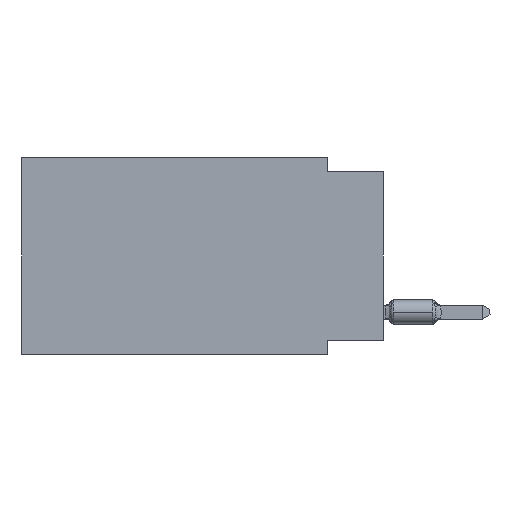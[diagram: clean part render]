
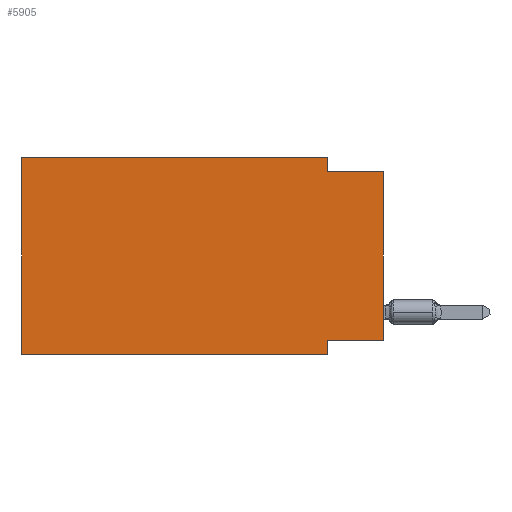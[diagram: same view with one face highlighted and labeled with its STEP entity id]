
A CAD part, left-side view. The second image highlights one B-rep face of the part: STEP entity #5905.
In plain terms, the highlighted planar face has unit normal (-1, 0, 0).
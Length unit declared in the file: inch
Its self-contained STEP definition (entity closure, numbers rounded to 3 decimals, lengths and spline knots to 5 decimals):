
#18 = LINE ( 'NONE', #9168, #2821 ) ;
#73 = CARTESIAN_POINT ( 'NONE',  ( 0., 0.1, 0. ) ) ;
#116 = DIRECTION ( 'NONE',  ( 0., 1., 0. ) ) ;
#189 = EDGE_CURVE ( 'NONE', #5356, #11744, #13301, .T. ) ;
#722 = VERTEX_POINT ( 'NONE', #19432 ) ;
#1417 = CARTESIAN_POINT ( 'NONE',  ( 0., 0., -0.025 ) ) ;
#1449 = EDGE_CURVE ( 'NONE', #10396, #11744, #18, .T. ) ;
#1761 = LINE ( 'NONE', #9203, #13726 ) ;
#1766 = EDGE_CURVE ( 'NONE', #18774, #15842, #13236, .T. ) ;
#2267 = AXIS2_PLACEMENT_3D ( 'NONE', #14849, #5990, #2820 ) ;
#2820 = DIRECTION ( 'NONE',  ( 0., 0., -1. ) ) ;
#2821 = VECTOR ( 'NONE', #16934, 39.37008 ) ;
#3088 = DIRECTION ( 'NONE',  ( 0., 0., -1. ) ) ;
#3176 = LINE ( 'NONE', #4674, #9659 ) ;
#3255 = VERTEX_POINT ( 'NONE', #12718 ) ;
#3363 = ORIENTED_EDGE ( 'NONE', *, *, #15018, .T. ) ;
#3401 = EDGE_CURVE ( 'NONE', #10396, #722, #13306, .T. ) ;
#4111 = ORIENTED_EDGE ( 'NONE', *, *, #7689, .F. ) ;
#4191 = ORIENTED_EDGE ( 'NONE', *, *, #189, .F. ) ;
#4222 = VECTOR ( 'NONE', #116, 39.37008 ) ;
#4353 = EDGE_LOOP ( 'NONE', ( #3363, #15088, #11310, #11307, #8534, #13548, #4191, #4111 ) ) ;
#4582 = CARTESIAN_POINT ( 'NONE',  ( 0., 0.1, -0.35 ) ) ;
#4674 = CARTESIAN_POINT ( 'NONE',  ( 0., 0.1, 0. ) ) ;
#5091 = VECTOR ( 'NONE', #12015, 39.37008 ) ;
#5356 = VERTEX_POINT ( 'NONE', #12535 ) ;
#5905 = ADVANCED_FACE ( 'NONE', ( #13651 ), #16355, .F. ) ;
#5990 = DIRECTION ( 'NONE',  ( 1., 0., 0. ) ) ;
#6943 = CARTESIAN_POINT ( 'NONE',  ( 0., 0.1, -0.025 ) ) ;
#7689 = EDGE_CURVE ( 'NONE', #3255, #5356, #11041, .T. ) ;
#8427 = DIRECTION ( 'NONE',  ( 0., 0., -1. ) ) ;
#8534 = ORIENTED_EDGE ( 'NONE', *, *, #3401, .F. ) ;
#8822 = CARTESIAN_POINT ( 'NONE',  ( 0., 0.1, -0.35 ) ) ;
#9168 = CARTESIAN_POINT ( 'NONE',  ( 0., 0.645, -0.35 ) ) ;
#9203 = CARTESIAN_POINT ( 'NONE',  ( 0., 0., 0. ) ) ;
#9493 = EDGE_CURVE ( 'NONE', #19387, #18774, #3176, .T. ) ;
#9659 = VECTOR ( 'NONE', #3088, 39.37008 ) ;
#9765 = CARTESIAN_POINT ( 'NONE',  ( 0., 0.645, -0.35 ) ) ;
#10012 = CARTESIAN_POINT ( 'NONE',  ( 0., 0.645, 0. ) ) ;
#10396 = VERTEX_POINT ( 'NONE', #9765 ) ;
#10439 = DIRECTION ( 'NONE',  ( 0., -1., 0. ) ) ;
#10609 = DIRECTION ( 'NONE',  ( 0., 0., 1. ) ) ;
#11041 = LINE ( 'NONE', #14120, #4222 ) ;
#11307 = ORIENTED_EDGE ( 'NONE', *, *, #16362, .F. ) ;
#11310 = ORIENTED_EDGE ( 'NONE', *, *, #9493, .F. ) ;
#11744 = VERTEX_POINT ( 'NONE', #4582 ) ;
#12015 = DIRECTION ( 'NONE',  ( 0., 0., 1. ) ) ;
#12033 = LINE ( 'NONE', #10012, #19112 ) ;
#12535 = CARTESIAN_POINT ( 'NONE',  ( 0., 0.1, -0.325 ) ) ;
#12718 = CARTESIAN_POINT ( 'NONE',  ( 0., 0., -0.325 ) ) ;
#13236 = LINE ( 'NONE', #15008, #13932 ) ;
#13301 = LINE ( 'NONE', #8822, #14770 ) ;
#13306 = LINE ( 'NONE', #19367, #5091 ) ;
#13548 = ORIENTED_EDGE ( 'NONE', *, *, #1449, .T. ) ;
#13651 = FACE_OUTER_BOUND ( 'NONE', #4353, .T. ) ;
#13726 = VECTOR ( 'NONE', #10609, 39.37008 ) ;
#13932 = VECTOR ( 'NONE', #10439, 39.37008 ) ;
#14120 = CARTESIAN_POINT ( 'NONE',  ( 0., 0., -0.325 ) ) ;
#14770 = VECTOR ( 'NONE', #8427, 39.37008 ) ;
#14849 = CARTESIAN_POINT ( 'NONE',  ( 0., 0.645, 0. ) ) ;
#15008 = CARTESIAN_POINT ( 'NONE',  ( 0., 0., -0.025 ) ) ;
#15018 = EDGE_CURVE ( 'NONE', #3255, #15842, #1761, .T. ) ;
#15088 = ORIENTED_EDGE ( 'NONE', *, *, #1766, .F. ) ;
#15842 = VERTEX_POINT ( 'NONE', #1417 ) ;
#16355 = PLANE ( 'NONE',  #2267 ) ;
#16362 = EDGE_CURVE ( 'NONE', #722, #19387, #12033, .T. ) ;
#16934 = DIRECTION ( 'NONE',  ( 0., -1., 0. ) ) ;
#18774 = VERTEX_POINT ( 'NONE', #6943 ) ;
#19112 = VECTOR ( 'NONE', #19257, 39.37008 ) ;
#19257 = DIRECTION ( 'NONE',  ( 0., -1., 0. ) ) ;
#19367 = CARTESIAN_POINT ( 'NONE',  ( 0., 0.645, 0. ) ) ;
#19387 = VERTEX_POINT ( 'NONE', #73 ) ;
#19432 = CARTESIAN_POINT ( 'NONE',  ( 0., 0.645, 0. ) ) ;
